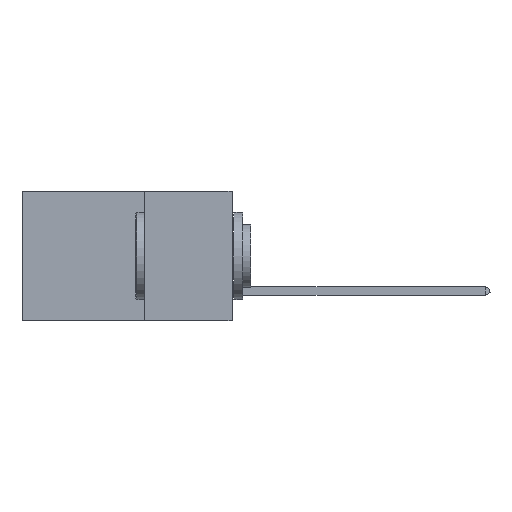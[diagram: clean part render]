
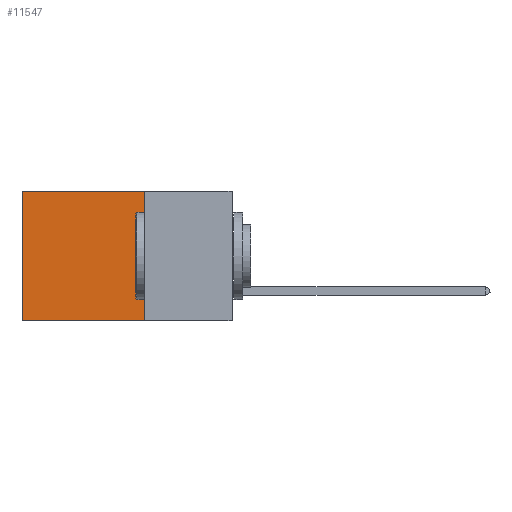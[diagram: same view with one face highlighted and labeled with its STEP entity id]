
A CAD part, left-side view. The second image highlights one B-rep face of the part: STEP entity #11547.
In plain terms, the highlighted planar face has unit normal (-1, 0, 0).
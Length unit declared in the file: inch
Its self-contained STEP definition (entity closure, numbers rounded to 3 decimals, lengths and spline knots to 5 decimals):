
#111 = CARTESIAN_POINT ( 'NONE',  ( 0.2875, 0.6, 0. ) ) ;
#1374 = CARTESIAN_POINT ( 'NONE',  ( 0.2875, 0.25, 0. ) ) ;
#2630 = VECTOR ( 'NONE', #7351, 39.37008 ) ;
#4822 = VERTEX_POINT ( 'NONE', #24183 ) ;
#6193 = DIRECTION ( 'NONE',  ( 0., 1., 0. ) ) ;
#7351 = DIRECTION ( 'NONE',  ( 0., 0., -1. ) ) ;
#9302 = DIRECTION ( 'NONE',  ( 1., 0., 0. ) ) ;
#9681 = VECTOR ( 'NONE', #13440, 39.37008 ) ;
#11547 = ADVANCED_FACE ( 'NONE', ( #28882 ), #17393, .F. ) ;
#12993 = CARTESIAN_POINT ( 'NONE',  ( 0.2875, 0.25, -0.37 ) ) ;
#13440 = DIRECTION ( 'NONE',  ( 0., 0., -1. ) ) ;
#14941 = ORIENTED_EDGE ( 'NONE', *, *, #28811, .T. ) ;
#15178 = VERTEX_POINT ( 'NONE', #12993 ) ;
#15315 = CARTESIAN_POINT ( 'NONE',  ( 0.2875, 0.6, 0. ) ) ;
#15399 = VECTOR ( 'NONE', #6193, 39.37008 ) ;
#16444 = LINE ( 'NONE', #15315, #2630 ) ;
#16779 = LINE ( 'NONE', #29533, #9681 ) ;
#17393 = PLANE ( 'NONE',  #24470 ) ;
#17535 = VECTOR ( 'NONE', #30406, 39.37008 ) ;
#17921 = EDGE_CURVE ( 'NONE', #4822, #15178, #16779, .T. ) ;
#18154 = CARTESIAN_POINT ( 'NONE',  ( 0.2875, 0.6, -0.37 ) ) ;
#19387 = EDGE_CURVE ( 'NONE', #15178, #27816, #31811, .T. ) ;
#19881 = EDGE_LOOP ( 'NONE', ( #30699, #21993, #26252, #14941 ) ) ;
#21265 = LINE ( 'NONE', #30881, #15399 ) ;
#21993 = ORIENTED_EDGE ( 'NONE', *, *, #19387, .F. ) ;
#22061 = EDGE_CURVE ( 'NONE', #27966, #27816, #16444, .T. ) ;
#22458 = DIRECTION ( 'NONE',  ( 0., 0., -1. ) ) ;
#24183 = CARTESIAN_POINT ( 'NONE',  ( 0.2875, 0.25, 0. ) ) ;
#24470 = AXIS2_PLACEMENT_3D ( 'NONE', #1374, #9302, #22458 ) ;
#26252 = ORIENTED_EDGE ( 'NONE', *, *, #17921, .F. ) ;
#27816 = VERTEX_POINT ( 'NONE', #18154 ) ;
#27966 = VERTEX_POINT ( 'NONE', #111 ) ;
#28811 = EDGE_CURVE ( 'NONE', #4822, #27966, #21265, .T. ) ;
#28882 = FACE_OUTER_BOUND ( 'NONE', #19881, .T. ) ;
#29533 = CARTESIAN_POINT ( 'NONE',  ( 0.2875, 0.25, 0. ) ) ;
#30406 = DIRECTION ( 'NONE',  ( 0., 1., 0. ) ) ;
#30699 = ORIENTED_EDGE ( 'NONE', *, *, #22061, .T. ) ;
#30881 = CARTESIAN_POINT ( 'NONE',  ( 0.2875, 0.25, 0. ) ) ;
#31811 = LINE ( 'NONE', #32407, #17535 ) ;
#32407 = CARTESIAN_POINT ( 'NONE',  ( 0.2875, 0.25, -0.37 ) ) ;
